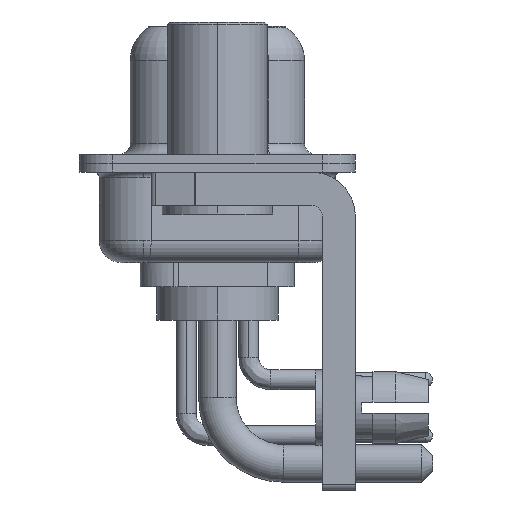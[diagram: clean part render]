
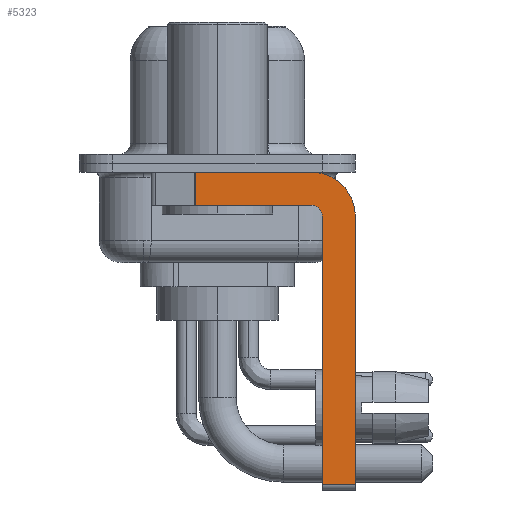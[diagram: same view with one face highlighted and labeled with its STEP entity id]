
A CAD part, left-side view. The second image highlights one B-rep face of the part: STEP entity #5323.
In plain terms, the highlighted planar face has unit normal (-1, 0, 0).
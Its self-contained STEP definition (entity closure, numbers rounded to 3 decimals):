
#50 = DIRECTION ( 'NONE',  ( 0., 0., -1. ) ) ;
#86 = DIRECTION ( 'NONE',  ( 0., -1., 0. ) ) ;
#524 = VECTOR ( 'NONE', #7966, 1000. ) ;
#581 = CIRCLE ( 'NONE', #19039, 2. ) ;
#875 = VERTEX_POINT ( 'NONE', #17276 ) ;
#881 = VECTOR ( 'NONE', #86, 1000. ) ;
#932 = CARTESIAN_POINT ( 'NONE',  ( -2.9, -6.25, -2.4 ) ) ;
#1106 = CARTESIAN_POINT ( 'NONE',  ( -2.9, 0.978, -1.9 ) ) ;
#1599 = DIRECTION ( 'NONE',  ( 1., 0., 0. ) ) ;
#1683 = CARTESIAN_POINT ( 'NONE',  ( -2.9, -6.25, -2.4 ) ) ;
#1895 = LINE ( 'NONE', #1683, #524 ) ;
#1921 = EDGE_CURVE ( 'NONE', #14123, #11239, #2305, .T. ) ;
#2141 = ORIENTED_EDGE ( 'NONE', *, *, #11509, .F. ) ;
#2166 = LINE ( 'NONE', #14691, #14821 ) ;
#2305 = LINE ( 'NONE', #11605, #10725 ) ;
#2504 = EDGE_CURVE ( 'NONE', #19443, #13865, #581, .T. ) ;
#2798 = DIRECTION ( 'NONE',  ( -1., 0., 0. ) ) ;
#2925 = EDGE_CURVE ( 'NONE', #18900, #11239, #15384, .T. ) ;
#3739 = ORIENTED_EDGE ( 'NONE', *, *, #15681, .T. ) ;
#3952 = EDGE_CURVE ( 'NONE', #7478, #14123, #11254, .T. ) ;
#4372 = ORIENTED_EDGE ( 'NONE', *, *, #1921, .F. ) ;
#4523 = CARTESIAN_POINT ( 'NONE',  ( -2.9, 3., -0.4 ) ) ;
#4921 = CARTESIAN_POINT ( 'NONE',  ( -2.9, -4.75, -2.4 ) ) ;
#5323 = ADVANCED_FACE ( 'NONE', ( #16087 ), #11407, .F. ) ;
#5394 = VERTEX_POINT ( 'NONE', #18951 ) ;
#5784 = CARTESIAN_POINT ( 'NONE',  ( -2.9, 0.978, -1.9 ) ) ;
#6405 = CARTESIAN_POINT ( 'NONE',  ( -2.9, 0.978, -0.4 ) ) ;
#7084 = ORIENTED_EDGE ( 'NONE', *, *, #3952, .F. ) ;
#7478 = VERTEX_POINT ( 'NONE', #4921 ) ;
#7513 = DIRECTION ( 'NONE',  ( 1., 0., 0. ) ) ;
#7622 = CARTESIAN_POINT ( 'NONE',  ( -2.9, -4.25, -2.4 ) ) ;
#7966 = DIRECTION ( 'NONE',  ( 0., 0., -1. ) ) ;
#8450 = DIRECTION ( 'NONE',  ( 0., -1., 0. ) ) ;
#8582 = DIRECTION ( 'NONE',  ( 0., 1., 0. ) ) ;
#8698 = CARTESIAN_POINT ( 'NONE',  ( -2.9, -4.75, -14.8 ) ) ;
#9087 = ORIENTED_EDGE ( 'NONE', *, *, #2925, .T. ) ;
#9378 = ORIENTED_EDGE ( 'NONE', *, *, #13219, .F. ) ;
#10725 = VECTOR ( 'NONE', #8582, 1000. ) ;
#11032 = CARTESIAN_POINT ( 'NONE',  ( -2.9, -4.25, -1.9 ) ) ;
#11239 = VERTEX_POINT ( 'NONE', #5784 ) ;
#11254 = CIRCLE ( 'NONE', #19175, 0.5 ) ;
#11407 = PLANE ( 'NONE',  #16032 ) ;
#11459 = CARTESIAN_POINT ( 'NONE',  ( -2.9, -4.25, -0.4 ) ) ;
#11509 = EDGE_CURVE ( 'NONE', #875, #7478, #16491, .T. ) ;
#11605 = CARTESIAN_POINT ( 'NONE',  ( -2.9, -4.25, -1.9 ) ) ;
#13219 = EDGE_CURVE ( 'NONE', #13865, #5394, #1895, .T. ) ;
#13410 = DIRECTION ( 'NONE',  ( 0., 0., -1. ) ) ;
#13865 = VERTEX_POINT ( 'NONE', #932 ) ;
#14003 = EDGE_CURVE ( 'NONE', #18900, #19443, #18686, .T. ) ;
#14123 = VERTEX_POINT ( 'NONE', #11032 ) ;
#14141 = VECTOR ( 'NONE', #13410, 1000. ) ;
#14691 = CARTESIAN_POINT ( 'NONE',  ( -2.9, -4.25, -14.55 ) ) ;
#14821 = VECTOR ( 'NONE', #8450, 1000. ) ;
#14935 = DIRECTION ( 'NONE',  ( 0., 0., 1. ) ) ;
#15105 = DIRECTION ( 'NONE',  ( 0., 0., -1. ) ) ;
#15384 = LINE ( 'NONE', #1106, #14141 ) ;
#15543 = ORIENTED_EDGE ( 'NONE', *, *, #2504, .F. ) ;
#15681 = EDGE_CURVE ( 'NONE', #875, #5394, #2166, .T. ) ;
#15863 = ORIENTED_EDGE ( 'NONE', *, *, #14003, .F. ) ;
#16032 = AXIS2_PLACEMENT_3D ( 'NONE', #17737, #1599, #50 ) ;
#16087 = FACE_OUTER_BOUND ( 'NONE', #16352, .T. ) ;
#16352 = EDGE_LOOP ( 'NONE', ( #15863, #9087, #4372, #7084, #2141, #3739, #9378, #15543 ) ) ;
#16491 = LINE ( 'NONE', #8698, #18931 ) ;
#16648 = CARTESIAN_POINT ( 'NONE',  ( -2.9, -4.25, -2.4 ) ) ;
#17067 = DIRECTION ( 'NONE',  ( 0., 0., 1. ) ) ;
#17276 = CARTESIAN_POINT ( 'NONE',  ( -2.9, -4.75, -14.55 ) ) ;
#17737 = CARTESIAN_POINT ( 'NONE',  ( -2.9, -4.25, -2.4 ) ) ;
#18686 = LINE ( 'NONE', #4523, #881 ) ;
#18900 = VERTEX_POINT ( 'NONE', #6405 ) ;
#18931 = VECTOR ( 'NONE', #14935, 1000. ) ;
#18951 = CARTESIAN_POINT ( 'NONE',  ( -2.9, -6.25, -14.55 ) ) ;
#19039 = AXIS2_PLACEMENT_3D ( 'NONE', #16648, #7513, #15105 ) ;
#19175 = AXIS2_PLACEMENT_3D ( 'NONE', #7622, #2798, #17067 ) ;
#19443 = VERTEX_POINT ( 'NONE', #11459 ) ;
